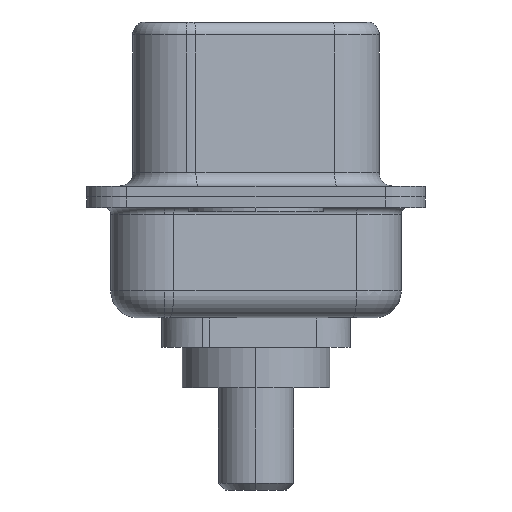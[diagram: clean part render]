
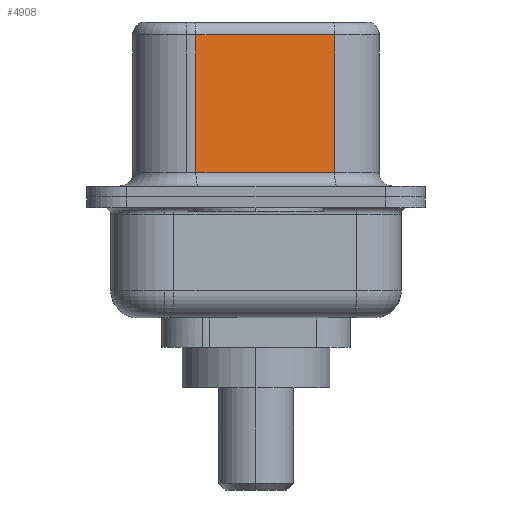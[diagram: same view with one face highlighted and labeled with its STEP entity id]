
A CAD part, left-side view. The second image highlights one B-rep face of the part: STEP entity #4908.
In plain terms, the highlighted planar face has unit normal (-0.985, -0.174, 0).
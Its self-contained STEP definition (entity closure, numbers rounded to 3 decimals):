
#36 = DIRECTION ( 'NONE',  ( -0.174, 0.985, 0. ) ) ;
#356 = LINE ( 'NONE', #757, #10921 ) ;
#424 = EDGE_LOOP ( 'NONE', ( #12745, #8508, #4219, #4534 ) ) ;
#433 = DIRECTION ( 'NONE',  ( 0.174, -0.985, 0. ) ) ;
#483 = LINE ( 'NONE', #4673, #3030 ) ;
#757 = CARTESIAN_POINT ( 'NONE',  ( 3.655, 2.233, 6.52 ) ) ;
#933 = CARTESIAN_POINT ( 'NONE',  ( 4.565, -2.927, 0.9 ) ) ;
#1268 = CARTESIAN_POINT ( 'NONE',  ( 4.565, -2.927, 6.52 ) ) ;
#1319 = PLANE ( 'NONE',  #2085 ) ;
#1332 = DIRECTION ( 'NONE',  ( 0.985, 0.174, 0. ) ) ;
#1484 = CARTESIAN_POINT ( 'NONE',  ( 4.565, -2.927, 6.52 ) ) ;
#2085 = AXIS2_PLACEMENT_3D ( 'NONE', #1484, #1332, #36 ) ;
#2192 = EDGE_CURVE ( 'NONE', #2796, #13596, #5223, .T. ) ;
#2403 = VECTOR ( 'NONE', #7011, 1000. ) ;
#2796 = VERTEX_POINT ( 'NONE', #11444 ) ;
#3030 = VECTOR ( 'NONE', #3655, 1000. ) ;
#3167 = LINE ( 'NONE', #12387, #10222 ) ;
#3655 = DIRECTION ( 'NONE',  ( -0.174, 0.985, 0. ) ) ;
#3686 = EDGE_CURVE ( 'NONE', #3827, #12371, #356, .T. ) ;
#3778 = DIRECTION ( 'NONE',  ( 0., 0., -1. ) ) ;
#3827 = VERTEX_POINT ( 'NONE', #6335 ) ;
#4219 = ORIENTED_EDGE ( 'NONE', *, *, #3686, .T. ) ;
#4534 = ORIENTED_EDGE ( 'NONE', *, *, #5767, .T. ) ;
#4673 = CARTESIAN_POINT ( 'NONE',  ( 4.565, -2.927, 6.02 ) ) ;
#4908 = ADVANCED_FACE ( 'NONE', ( #5522 ), #1319, .F. ) ;
#5223 = LINE ( 'NONE', #1268, #2403 ) ;
#5522 = FACE_OUTER_BOUND ( 'NONE', #424, .T. ) ;
#5767 = EDGE_CURVE ( 'NONE', #12371, #13596, #3167, .T. ) ;
#6335 = CARTESIAN_POINT ( 'NONE',  ( 3.655, 2.233, 6.02 ) ) ;
#7011 = DIRECTION ( 'NONE',  ( 0., 0., -1. ) ) ;
#8508 = ORIENTED_EDGE ( 'NONE', *, *, #13378, .T. ) ;
#8640 = CARTESIAN_POINT ( 'NONE',  ( 3.655, 2.233, 0.9 ) ) ;
#10222 = VECTOR ( 'NONE', #433, 1000. ) ;
#10921 = VECTOR ( 'NONE', #3778, 1000. ) ;
#11444 = CARTESIAN_POINT ( 'NONE',  ( 4.565, -2.927, 6.02 ) ) ;
#12371 = VERTEX_POINT ( 'NONE', #8640 ) ;
#12387 = CARTESIAN_POINT ( 'NONE',  ( 4.565, -2.927, 0.9 ) ) ;
#12745 = ORIENTED_EDGE ( 'NONE', *, *, #2192, .F. ) ;
#13378 = EDGE_CURVE ( 'NONE', #2796, #3827, #483, .T. ) ;
#13596 = VERTEX_POINT ( 'NONE', #933 ) ;
